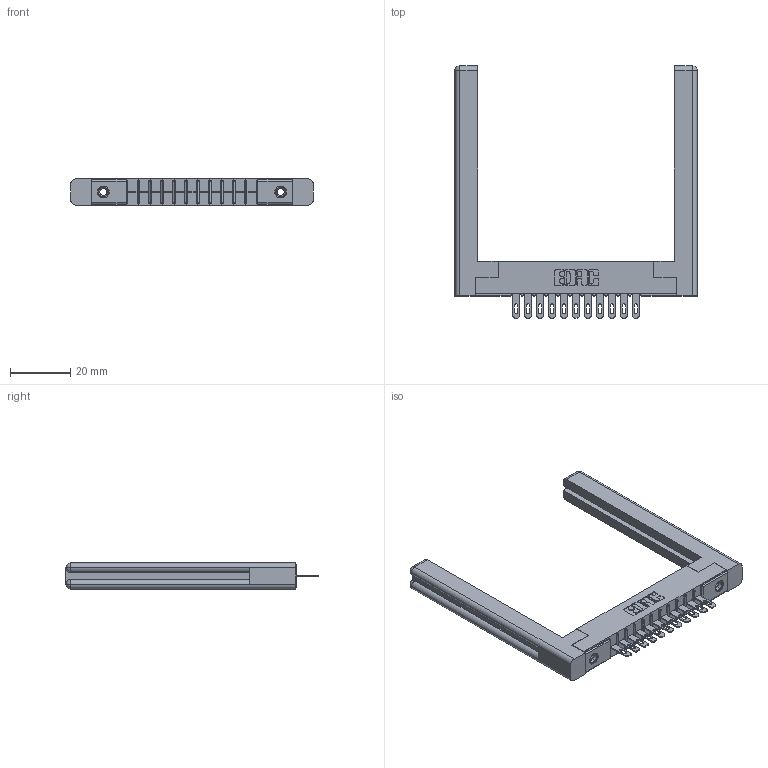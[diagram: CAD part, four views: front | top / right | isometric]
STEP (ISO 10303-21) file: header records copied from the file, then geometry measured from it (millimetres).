
FILE_DESCRIPTION (( 'STEP AP203' ), '1' );
FILE_NAME ('356-011-400-158.STEP', '2020-09-23T10:18:22', ( '' ), ( '' ), 'SwSTEP 2.0', 'SolidWorks 2020', '' );
FILE_SCHEMA (( 'CONFIG_CONTROL_DESIGN' ));
Length unit declared in the file: inch
Products named in the file (5): 307-220-058; 356-011-400-158; 306-290-001_100; 345-250-001_345-250-001-102; 306 Part_.156 Dia
Assembly tree (16 placements, depth 2):
  356-011-400-158
    306 Part_.156 Dia
    306-290-001_100  x11
    345-250-001_345-250-001-102  x2
    307-220-058  x2
Bounding box: 80.21 x 83.52 x 8.71 mm (x, y, z)
Volume: 13114.8 mm3; surface area: 13214.1 mm2
Topology: 16 solids, 16 shells, 1094 faces, 3035 edges, 1950 vertices
Faces by surface type: plane 702, cylinder 324, sphere 44, cone 12, torus 12
Entity records: 17071 total; most frequent: CARTESIAN_POINT 2871, DIRECTION 2790, ORIENTED_EDGE 2784, EDGE_CURVE 1392, LINE 1064, VECTOR 1064, VERTEX_POINT 890, AXIS2_PLACEMENT_3D 863
